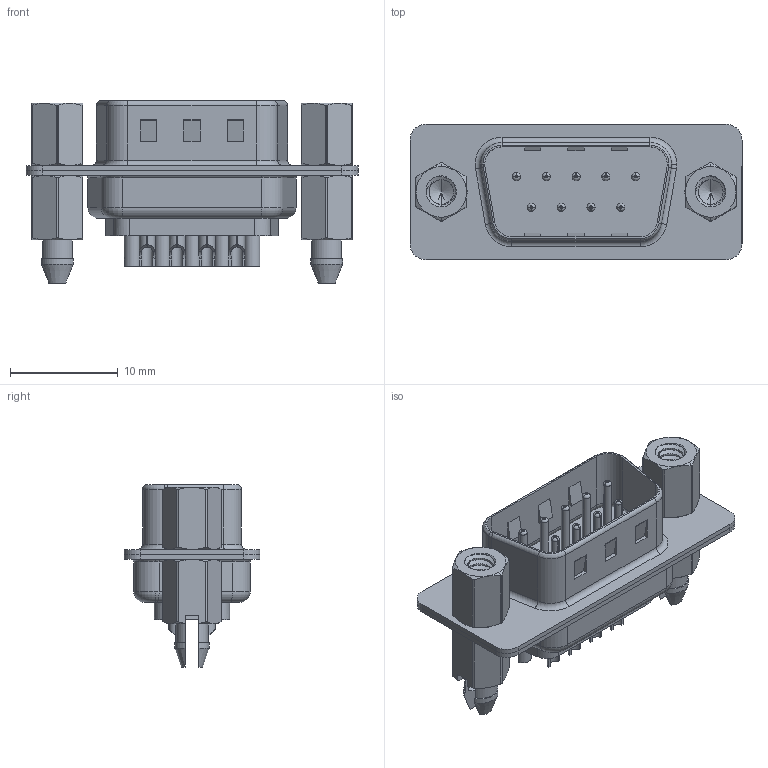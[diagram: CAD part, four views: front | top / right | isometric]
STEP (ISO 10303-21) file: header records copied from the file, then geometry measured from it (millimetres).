
FILE_DESCRIPTION (( 'STEP AP203' ), '1' );
FILE_NAME ('627-009-222-067.STEP', '2020-07-13T23:18:56', ( '' ), ( '' ), 'SwSTEP 2.0', 'SolidWorks 2020', '' );
FILE_SCHEMA (( 'CONFIG_CONTROL_DESIGN' ));
Length unit declared in the file: millimetre
Products named in the file (8): 627 Contact Row 2_22L; 627 Housing_09 LP; 627-009-222-067; 627 Shell Front_09 Contacts; 627 Contact Row 1_22L; 627 4-40 Threaded Boardlock_LP; 627 4-40 Hex Standoff; 627 Shell Rear_09 Contacts
Assembly tree (16 placements, depth 2):
  627-009-222-067
    627 Housing_09 LP
    627 Shell Front_09 Contacts
    627 Shell Rear_09 Contacts
    627 Contact Row 1_22L  x5
    627 Contact Row 2_22L  x4
    627 4-40 Hex Standoff  x2
    627 4-40 Threaded Boardlock_LP  x2
Bounding box: 30.8 x 12.6 x 16.9 mm (x, y, z)
Volume: 1642.3 mm3; surface area: 4726.9 mm2
Topology: 16 solids, 16 shells, 1080 faces, 2813 edges, 1792 vertices
Faces by surface type: cylinder 494, plane 287, torus 245, cone 36, bspline 18
Entity records: 21982 total; most frequent: CARTESIAN_POINT 7325, DIRECTION 2949, ORIENTED_EDGE 2836, EDGE_CURVE 1418, AXIS2_PLACEMENT_3D 1170, VERTEX_POINT 905, EDGE_LOOP 627, VECTOR 609
